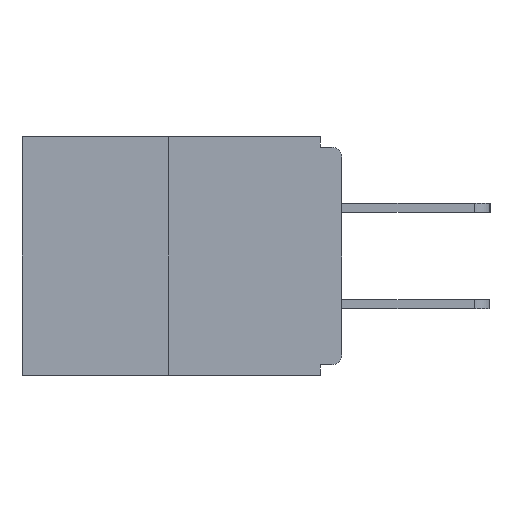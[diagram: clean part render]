
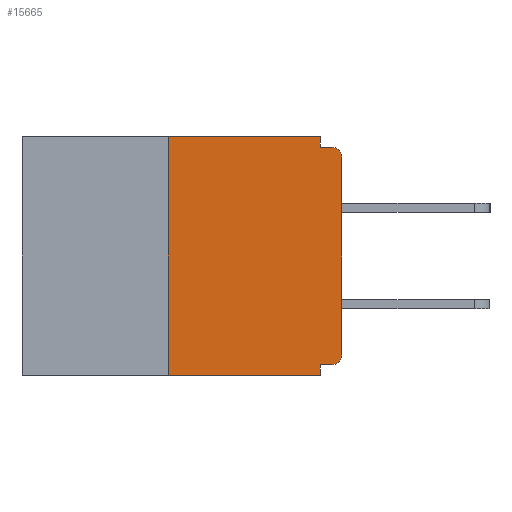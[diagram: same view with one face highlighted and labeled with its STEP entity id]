
A CAD part, left-side view. The second image highlights one B-rep face of the part: STEP entity #15665.
In plain terms, the highlighted planar face has unit normal (-1, 0, 0).
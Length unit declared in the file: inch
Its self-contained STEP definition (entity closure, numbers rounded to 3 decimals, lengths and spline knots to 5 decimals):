
#48 = LINE ( 'NONE', #7864, #11719 ) ;
#187 = EDGE_CURVE ( 'NONE', #9382, #2420, #4159, .T. ) ;
#216 = DIRECTION ( 'NONE',  ( 0., 0., 1. ) ) ;
#314 = AXIS2_PLACEMENT_3D ( 'NONE', #7923, #16928, #3943 ) ;
#325 = DIRECTION ( 'NONE',  ( 1., 0., 0. ) ) ;
#1331 = VERTEX_POINT ( 'NONE', #12213 ) ;
#1386 = LINE ( 'NONE', #2888, #6107 ) ;
#1510 = EDGE_LOOP ( 'NONE', ( #2875, #10373, #1874, #6229, #4945, #14607, #7341, #16556, #12957, #13508 ) ) ;
#1820 = CARTESIAN_POINT ( 'NONE',  ( 0., 0.015, -0.313 ) ) ;
#1874 = ORIENTED_EDGE ( 'NONE', *, *, #5010, .T. ) ;
#2420 = VERTEX_POINT ( 'NONE', #13750 ) ;
#2604 = DIRECTION ( 'NONE',  ( 0., 0., -1. ) ) ;
#2875 = ORIENTED_EDGE ( 'NONE', *, *, #5428, .F. ) ;
#2888 = CARTESIAN_POINT ( 'NONE',  ( 0., 0.46, -0.343 ) ) ;
#3045 = CARTESIAN_POINT ( 'NONE',  ( 0., 0.031, -0.328 ) ) ;
#3140 = LINE ( 'NONE', #15463, #3947 ) ;
#3189 = LINE ( 'NONE', #6559, #16901 ) ;
#3366 = DIRECTION ( 'NONE',  ( 0., -1., 0. ) ) ;
#3816 = AXIS2_PLACEMENT_3D ( 'NONE', #10545, #325, #9533 ) ;
#3865 = VECTOR ( 'NONE', #216, 39.37008 ) ;
#3943 = DIRECTION ( 'NONE',  ( 0., 0., -1. ) ) ;
#3947 = VECTOR ( 'NONE', #9034, 39.37008 ) ;
#4100 = CARTESIAN_POINT ( 'NONE',  ( 0., 0.25, 0. ) ) ;
#4159 = LINE ( 'NONE', #10015, #14602 ) ;
#4447 = CARTESIAN_POINT ( 'NONE',  ( 0., 0.015, -0.015 ) ) ;
#4536 = CARTESIAN_POINT ( 'NONE',  ( 0., 0.031, -0.343 ) ) ;
#4541 = AXIS2_PLACEMENT_3D ( 'NONE', #1820, #13535, #8713 ) ;
#4564 = CARTESIAN_POINT ( 'NONE',  ( 0., 0.46, 0. ) ) ;
#4706 = CIRCLE ( 'NONE', #314, 0.015 ) ;
#4891 = EDGE_CURVE ( 'NONE', #10718, #10656, #11885, .T. ) ;
#4926 = CARTESIAN_POINT ( 'NONE',  ( 0., 0., -0.313 ) ) ;
#4945 = ORIENTED_EDGE ( 'NONE', *, *, #15340, .F. ) ;
#5010 = EDGE_CURVE ( 'NONE', #10718, #10394, #1386, .T. ) ;
#5269 = LINE ( 'NONE', #4564, #13679 ) ;
#5428 = EDGE_CURVE ( 'NONE', #10656, #12507, #5269, .T. ) ;
#6107 = VECTOR ( 'NONE', #8376, 39.37008 ) ;
#6211 = CIRCLE ( 'NONE', #4541, 0.015 ) ;
#6229 = ORIENTED_EDGE ( 'NONE', *, *, #15030, .F. ) ;
#6282 = DIRECTION ( 'NONE',  ( 0., 0., 1. ) ) ;
#6559 = CARTESIAN_POINT ( 'NONE',  ( 0., 0.031, 0. ) ) ;
#6602 = CARTESIAN_POINT ( 'NONE',  ( 0., 0.25, 0. ) ) ;
#7011 = DIRECTION ( 'NONE',  ( 0., 1., 0. ) ) ;
#7341 = ORIENTED_EDGE ( 'NONE', *, *, #187, .T. ) ;
#7864 = CARTESIAN_POINT ( 'NONE',  ( 0., 0.031, -0.343 ) ) ;
#7923 = CARTESIAN_POINT ( 'NONE',  ( 0., 0.015, -0.03 ) ) ;
#8376 = DIRECTION ( 'NONE',  ( 0., -1., 0. ) ) ;
#8478 = CARTESIAN_POINT ( 'NONE',  ( 0., 0., -0.328 ) ) ;
#8713 = DIRECTION ( 'NONE',  ( 0., 0., -1. ) ) ;
#8979 = CARTESIAN_POINT ( 'NONE',  ( 0., 0.031, 0. ) ) ;
#9034 = DIRECTION ( 'NONE',  ( 0., -1., 0. ) ) ;
#9382 = VERTEX_POINT ( 'NONE', #4926 ) ;
#9533 = DIRECTION ( 'NONE',  ( 0., 0., -1. ) ) ;
#10015 = CARTESIAN_POINT ( 'NONE',  ( 0., 0., 0. ) ) ;
#10373 = ORIENTED_EDGE ( 'NONE', *, *, #4891, .F. ) ;
#10394 = VERTEX_POINT ( 'NONE', #4536 ) ;
#10545 = CARTESIAN_POINT ( 'NONE',  ( 0., 0.46, 0. ) ) ;
#10656 = VERTEX_POINT ( 'NONE', #4100 ) ;
#10718 = VERTEX_POINT ( 'NONE', #16359 ) ;
#10845 = CARTESIAN_POINT ( 'NONE',  ( 0., 0.015, -0.328 ) ) ;
#11704 = EDGE_CURVE ( 'NONE', #12507, #1331, #3189, .T. ) ;
#11719 = VECTOR ( 'NONE', #2604, 39.37008 ) ;
#11885 = LINE ( 'NONE', #6602, #3865 ) ;
#12143 = PLANE ( 'NONE',  #3816 ) ;
#12213 = CARTESIAN_POINT ( 'NONE',  ( 0., 0.031, -0.015 ) ) ;
#12319 = FACE_OUTER_BOUND ( 'NONE', #1510, .T. ) ;
#12420 = EDGE_CURVE ( 'NONE', #12715, #9382, #6211, .T. ) ;
#12507 = VERTEX_POINT ( 'NONE', #8979 ) ;
#12715 = VERTEX_POINT ( 'NONE', #10845 ) ;
#12833 = VERTEX_POINT ( 'NONE', #4447 ) ;
#12957 = ORIENTED_EDGE ( 'NONE', *, *, #13289, .F. ) ;
#13289 = EDGE_CURVE ( 'NONE', #1331, #12833, #3140, .T. ) ;
#13508 = ORIENTED_EDGE ( 'NONE', *, *, #11704, .F. ) ;
#13535 = DIRECTION ( 'NONE',  ( -1., 0., 0. ) ) ;
#13679 = VECTOR ( 'NONE', #3366, 39.37008 ) ;
#13750 = CARTESIAN_POINT ( 'NONE',  ( 0., 0., -0.03 ) ) ;
#13905 = LINE ( 'NONE', #8478, #14313 ) ;
#14313 = VECTOR ( 'NONE', #7011, 39.37008 ) ;
#14602 = VECTOR ( 'NONE', #6282, 39.37008 ) ;
#14607 = ORIENTED_EDGE ( 'NONE', *, *, #12420, .T. ) ;
#15030 = EDGE_CURVE ( 'NONE', #15347, #10394, #48, .T. ) ;
#15340 = EDGE_CURVE ( 'NONE', #12715, #15347, #13905, .T. ) ;
#15347 = VERTEX_POINT ( 'NONE', #3045 ) ;
#15458 = EDGE_CURVE ( 'NONE', #2420, #12833, #4706, .T. ) ;
#15463 = CARTESIAN_POINT ( 'NONE',  ( 0., 0., -0.015 ) ) ;
#15665 = ADVANCED_FACE ( 'NONE', ( #12319 ), #12143, .F. ) ;
#16095 = DIRECTION ( 'NONE',  ( 0., 0., -1. ) ) ;
#16359 = CARTESIAN_POINT ( 'NONE',  ( 0., 0.25, -0.343 ) ) ;
#16556 = ORIENTED_EDGE ( 'NONE', *, *, #15458, .T. ) ;
#16901 = VECTOR ( 'NONE', #16095, 39.37008 ) ;
#16928 = DIRECTION ( 'NONE',  ( -1., 0., 0. ) ) ;
